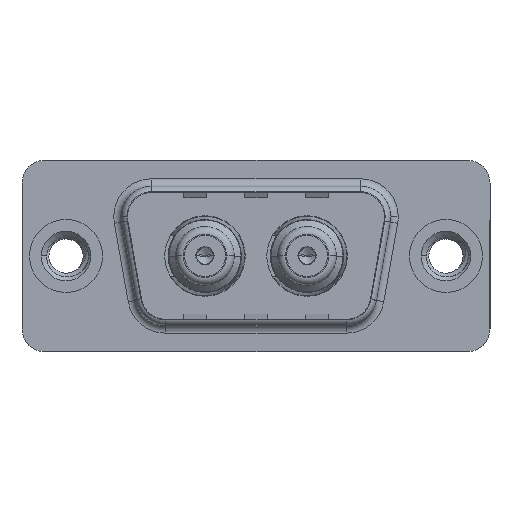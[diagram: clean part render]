
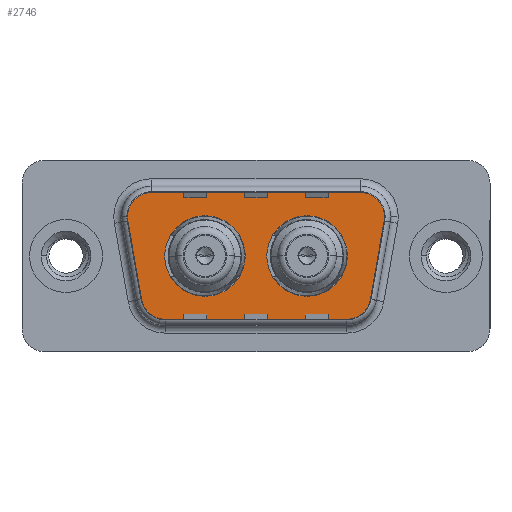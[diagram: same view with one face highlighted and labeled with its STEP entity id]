
A CAD part, top view. The second image highlights one B-rep face of the part: STEP entity #2746.
In plain terms, the highlighted planar face has unit normal (0, 0, 1).
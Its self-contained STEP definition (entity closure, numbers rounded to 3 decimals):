
#11 = DIRECTION ( 'NONE',  ( 0.174, -0.985, 0. ) ) ;
#209 = CIRCLE ( 'NONE', #12725, 2.65 ) ;
#293 = ORIENTED_EDGE ( 'NONE', *, *, #13277, .T. ) ;
#502 = AXIS2_PLACEMENT_3D ( 'NONE', #576, #8512, #1692 ) ;
#517 = VERTEX_POINT ( 'NONE', #4848 ) ;
#574 = ORIENTED_EDGE ( 'NONE', *, *, #12013, .T. ) ;
#576 = CARTESIAN_POINT ( 'NONE',  ( 9.14, 0., 0. ) ) ;
#756 = VERTEX_POINT ( 'NONE', #13458 ) ;
#896 = CARTESIAN_POINT ( 'NONE',  ( 6.459, -4.9, 0. ) ) ;
#1001 = CARTESIAN_POINT ( 'NONE',  ( 18.541, -4.9, 0. ) ) ;
#1124 = VECTOR ( 'NONE', #7388, 1000. ) ;
#1169 = AXIS2_PLACEMENT_3D ( 'NONE', #3155, #10948, #4972 ) ;
#1239 = DIRECTION ( 'NONE',  ( 1., 0., 0. ) ) ;
#1328 = VECTOR ( 'NONE', #12120, 1000. ) ;
#1432 = DIRECTION ( 'NONE',  ( 0., 0., 1. ) ) ;
#1486 = VERTEX_POINT ( 'NONE', #9844 ) ;
#1545 = EDGE_CURVE ( 'NONE', #756, #13352, #8998, .T. ) ;
#1692 = DIRECTION ( 'NONE',  ( 1., 0., 0. ) ) ;
#1739 = VERTEX_POINT ( 'NONE', #5764 ) ;
#1873 = CARTESIAN_POINT ( 'NONE',  ( 20.511, -3.247, 0. ) ) ;
#1970 = PLANE ( 'NONE',  #3819 ) ;
#1998 = CARTESIAN_POINT ( 'NONE',  ( 15.86, 0., 0. ) ) ;
#2015 = DIRECTION ( 'NONE',  ( 0., 0., 1. ) ) ;
#2183 = VECTOR ( 'NONE', #4169, 1000. ) ;
#2216 = CARTESIAN_POINT ( 'NONE',  ( 18.541, -2.9, 0. ) ) ;
#2591 = CARTESIAN_POINT ( 'NONE',  ( 21.534, 2.553, 0. ) ) ;
#2605 = EDGE_CURVE ( 'NONE', #8238, #13891, #14224, .T. ) ;
#2650 = DIRECTION ( 'NONE',  ( 0., 0., 1. ) ) ;
#2746 = ADVANCED_FACE ( 'NONE', ( #5578, #12067, #11354 ), #1970, .T. ) ;
#2965 = DIRECTION ( 'NONE',  ( 0., 0., 1. ) ) ;
#3095 = DIRECTION ( 'NONE',  ( 0., 0., 1. ) ) ;
#3108 = DIRECTION ( 'NONE',  ( 1., 0., 0. ) ) ;
#3155 = CARTESIAN_POINT ( 'NONE',  ( 6.459, -2.9, 0. ) ) ;
#3216 = ORIENTED_EDGE ( 'NONE', *, *, #7741, .T. ) ;
#3314 = EDGE_CURVE ( 'NONE', #13352, #5946, #14367, .T. ) ;
#3429 = EDGE_CURVE ( 'NONE', #9078, #10015, #7158, .T. ) ;
#3819 = AXIS2_PLACEMENT_3D ( 'NONE', #2216, #1432, #1239 ) ;
#3895 = CARTESIAN_POINT ( 'NONE',  ( 18.541, -2.9, 0. ) ) ;
#4019 = VERTEX_POINT ( 'NONE', #13559 ) ;
#4169 = DIRECTION ( 'NONE',  ( 1., 0., 0. ) ) ;
#4418 = CIRCLE ( 'NONE', #10946, 2. ) ;
#4848 = CARTESIAN_POINT ( 'NONE',  ( 6.49, 0., 0. ) ) ;
#4896 = ORIENTED_EDGE ( 'NONE', *, *, #8299, .F. ) ;
#4960 = CIRCLE ( 'NONE', #502, 2.65 ) ;
#4972 = DIRECTION ( 'NONE',  ( -1., 0., 0. ) ) ;
#5578 = FACE_BOUND ( 'NONE', #7682, .T. ) ;
#5584 = ORIENTED_EDGE ( 'NONE', *, *, #3429, .T. ) ;
#5657 = DIRECTION ( 'NONE',  ( 0., 0., 1. ) ) ;
#5764 = CARTESIAN_POINT ( 'NONE',  ( 13.21, 0., 0. ) ) ;
#5946 = VERTEX_POINT ( 'NONE', #1001 ) ;
#6200 = EDGE_CURVE ( 'NONE', #5946, #8238, #7496, .T. ) ;
#6221 = EDGE_CURVE ( 'NONE', #1486, #9078, #10245, .T. ) ;
#6339 = DIRECTION ( 'NONE',  ( -1., 0., 0. ) ) ;
#6448 = EDGE_CURVE ( 'NONE', #8847, #1739, #14520, .T. ) ;
#6762 = CARTESIAN_POINT ( 'NONE',  ( 3.466, 2.553, 0. ) ) ;
#7109 = ORIENTED_EDGE ( 'NONE', *, *, #3314, .T. ) ;
#7158 = LINE ( 'NONE', #13371, #1124 ) ;
#7365 = EDGE_LOOP ( 'NONE', ( #4896, #13169 ) ) ;
#7388 = DIRECTION ( 'NONE',  ( -1., 0., 0. ) ) ;
#7447 = AXIS2_PLACEMENT_3D ( 'NONE', #3895, #3095, #12399 ) ;
#7477 = DIRECTION ( 'NONE',  ( 1., 0., 0. ) ) ;
#7496 = CIRCLE ( 'NONE', #7447, 2. ) ;
#7682 = EDGE_LOOP ( 'NONE', ( #9191, #10847 ) ) ;
#7741 = EDGE_CURVE ( 'NONE', #13891, #1486, #9660, .T. ) ;
#7980 = CIRCLE ( 'NONE', #13734, 2.65 ) ;
#8062 = VERTEX_POINT ( 'NONE', #11915 ) ;
#8238 = VERTEX_POINT ( 'NONE', #1873 ) ;
#8299 = EDGE_CURVE ( 'NONE', #8062, #517, #209, .T. ) ;
#8512 = DIRECTION ( 'NONE',  ( 0., 0., 1. ) ) ;
#8718 = AXIS2_PLACEMENT_3D ( 'NONE', #13336, #2965, #7477 ) ;
#8795 = CARTESIAN_POINT ( 'NONE',  ( 21.534, 2.553, 0. ) ) ;
#8837 = CARTESIAN_POINT ( 'NONE',  ( 9.14, 0., 0. ) ) ;
#8847 = VERTEX_POINT ( 'NONE', #14238 ) ;
#8995 = DIRECTION ( 'NONE',  ( 0., 0., 1. ) ) ;
#8998 = CIRCLE ( 'NONE', #1169, 2. ) ;
#9078 = VERTEX_POINT ( 'NONE', #9347 ) ;
#9191 = ORIENTED_EDGE ( 'NONE', *, *, #6448, .F. ) ;
#9347 = CARTESIAN_POINT ( 'NONE',  ( 19.564, 4.9, 0. ) ) ;
#9511 = CARTESIAN_POINT ( 'NONE',  ( 5.436, 2.9, 0. ) ) ;
#9563 = CARTESIAN_POINT ( 'NONE',  ( 6.459, -4.9, 0. ) ) ;
#9660 = CIRCLE ( 'NONE', #12511, 2. ) ;
#9844 = CARTESIAN_POINT ( 'NONE',  ( 21.564, 2.9, 0. ) ) ;
#10002 = DIRECTION ( 'NONE',  ( 0., 0., 1. ) ) ;
#10015 = VERTEX_POINT ( 'NONE', #11205 ) ;
#10023 = DIRECTION ( 'NONE',  ( 1., 0., 0. ) ) ;
#10143 = LINE ( 'NONE', #6762, #10518 ) ;
#10245 = CIRCLE ( 'NONE', #12105, 2. ) ;
#10518 = VECTOR ( 'NONE', #11, 1000. ) ;
#10632 = ORIENTED_EDGE ( 'NONE', *, *, #2605, .T. ) ;
#10688 = DIRECTION ( 'NONE',  ( 1., 0., 0. ) ) ;
#10847 = ORIENTED_EDGE ( 'NONE', *, *, #13571, .F. ) ;
#10946 = AXIS2_PLACEMENT_3D ( 'NONE', #9511, #2650, #10688 ) ;
#10948 = DIRECTION ( 'NONE',  ( 0., 0., 1. ) ) ;
#11067 = EDGE_CURVE ( 'NONE', #517, #8062, #4960, .T. ) ;
#11084 = CARTESIAN_POINT ( 'NONE',  ( 19.564, 2.9, 0. ) ) ;
#11205 = CARTESIAN_POINT ( 'NONE',  ( 5.436, 4.9, 0. ) ) ;
#11354 = FACE_OUTER_BOUND ( 'NONE', #12592, .T. ) ;
#11915 = CARTESIAN_POINT ( 'NONE',  ( 11.79, 0., 0. ) ) ;
#12013 = EDGE_CURVE ( 'NONE', #4019, #756, #10143, .T. ) ;
#12067 = FACE_BOUND ( 'NONE', #7365, .T. ) ;
#12105 = AXIS2_PLACEMENT_3D ( 'NONE', #11084, #8995, #6339 ) ;
#12120 = DIRECTION ( 'NONE',  ( 0.174, 0.985, 0. ) ) ;
#12399 = DIRECTION ( 'NONE',  ( 1., 0., 0. ) ) ;
#12511 = AXIS2_PLACEMENT_3D ( 'NONE', #12550, #5657, #13716 ) ;
#12550 = CARTESIAN_POINT ( 'NONE',  ( 19.564, 2.9, 0. ) ) ;
#12592 = EDGE_LOOP ( 'NONE', ( #14374, #10632, #3216, #13886, #5584, #293, #574, #14324, #7109 ) ) ;
#12725 = AXIS2_PLACEMENT_3D ( 'NONE', #8837, #2015, #10023 ) ;
#13169 = ORIENTED_EDGE ( 'NONE', *, *, #11067, .F. ) ;
#13277 = EDGE_CURVE ( 'NONE', #10015, #4019, #4418, .T. ) ;
#13336 = CARTESIAN_POINT ( 'NONE',  ( 15.86, 0., 0. ) ) ;
#13352 = VERTEX_POINT ( 'NONE', #9563 ) ;
#13371 = CARTESIAN_POINT ( 'NONE',  ( 5.436, 4.9, 0. ) ) ;
#13458 = CARTESIAN_POINT ( 'NONE',  ( 4.489, -3.247, 0. ) ) ;
#13559 = CARTESIAN_POINT ( 'NONE',  ( 3.466, 2.553, 0. ) ) ;
#13571 = EDGE_CURVE ( 'NONE', #1739, #8847, #7980, .T. ) ;
#13716 = DIRECTION ( 'NONE',  ( -1., 0., 0. ) ) ;
#13734 = AXIS2_PLACEMENT_3D ( 'NONE', #1998, #10002, #3108 ) ;
#13886 = ORIENTED_EDGE ( 'NONE', *, *, #6221, .T. ) ;
#13891 = VERTEX_POINT ( 'NONE', #2591 ) ;
#14224 = LINE ( 'NONE', #8795, #1328 ) ;
#14238 = CARTESIAN_POINT ( 'NONE',  ( 18.51, 0., 0. ) ) ;
#14324 = ORIENTED_EDGE ( 'NONE', *, *, #1545, .T. ) ;
#14367 = LINE ( 'NONE', #896, #2183 ) ;
#14374 = ORIENTED_EDGE ( 'NONE', *, *, #6200, .T. ) ;
#14520 = CIRCLE ( 'NONE', #8718, 2.65 ) ;
